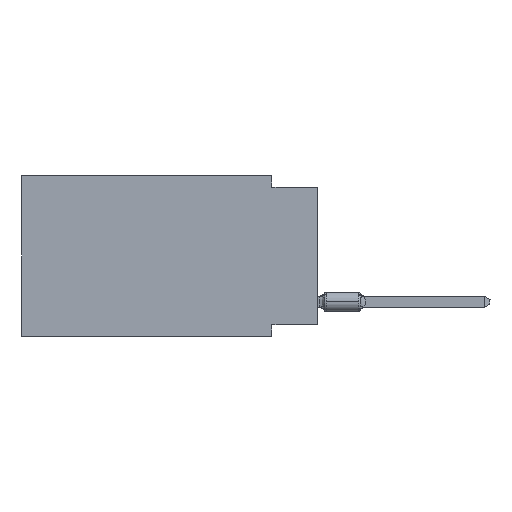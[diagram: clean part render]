
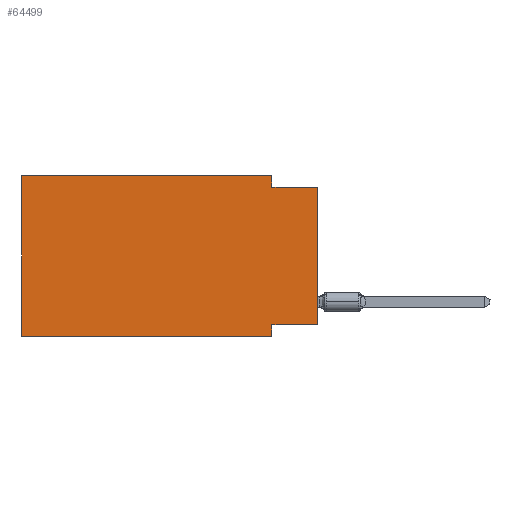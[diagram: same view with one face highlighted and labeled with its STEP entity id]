
A CAD part, left-side view. The second image highlights one B-rep face of the part: STEP entity #64499.
In plain terms, the highlighted planar face has unit normal (-1, 0, 0).
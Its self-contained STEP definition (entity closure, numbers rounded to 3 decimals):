
#1367 = CARTESIAN_POINT ( 'NONE',  ( 0., 16.383, 0. ) ) ;
#1848 = CARTESIAN_POINT ( 'NONE',  ( 0., 16.383, 0. ) ) ;
#3605 = VECTOR ( 'NONE', #41586, 1000. ) ;
#5541 = ORIENTED_EDGE ( 'NONE', *, *, #23059, .T. ) ;
#5818 = LINE ( 'NONE', #66674, #12349 ) ;
#6255 = LINE ( 'NONE', #52389, #24278 ) ;
#6706 = DIRECTION ( 'NONE',  ( 0., 0., 1. ) ) ;
#9025 = CARTESIAN_POINT ( 'NONE',  ( 0., 2.54, 0. ) ) ;
#10659 = EDGE_CURVE ( 'NONE', #60522, #26659, #27059, .T. ) ;
#12349 = VECTOR ( 'NONE', #78007, 1000. ) ;
#13057 = LINE ( 'NONE', #60876, #57707 ) ;
#13425 = VECTOR ( 'NONE', #55308, 1000. ) ;
#15426 = CARTESIAN_POINT ( 'NONE',  ( 0., 0., -8.255 ) ) ;
#16451 = ORIENTED_EDGE ( 'NONE', *, *, #61901, .F. ) ;
#17697 = CARTESIAN_POINT ( 'NONE',  ( 0., 16.383, 0. ) ) ;
#18842 = EDGE_CURVE ( 'NONE', #26659, #22340, #69042, .T. ) ;
#20145 = DIRECTION ( 'NONE',  ( 0., -1., 0. ) ) ;
#22340 = VERTEX_POINT ( 'NONE', #9025 ) ;
#23059 = EDGE_CURVE ( 'NONE', #24144, #85469, #40211, .T. ) ;
#24144 = VERTEX_POINT ( 'NONE', #15426 ) ;
#24278 = VECTOR ( 'NONE', #20145, 1000. ) ;
#26659 = VERTEX_POINT ( 'NONE', #17697 ) ;
#27059 = LINE ( 'NONE', #1367, #13425 ) ;
#28385 = FACE_OUTER_BOUND ( 'NONE', #82070, .T. ) ;
#29486 = CARTESIAN_POINT ( 'NONE',  ( 0., 16.383, 0. ) ) ;
#30424 = EDGE_CURVE ( 'NONE', #35867, #85469, #6255, .T. ) ;
#33253 = CARTESIAN_POINT ( 'NONE',  ( 0., 0., 0. ) ) ;
#35867 = VERTEX_POINT ( 'NONE', #68043 ) ;
#36164 = EDGE_CURVE ( 'NONE', #22340, #35867, #5818, .T. ) ;
#40178 = PLANE ( 'NONE',  #59316 ) ;
#40211 = LINE ( 'NONE', #33253, #54116 ) ;
#41586 = DIRECTION ( 'NONE',  ( 0., 1., 0. ) ) ;
#42982 = DIRECTION ( 'NONE',  ( 0., -1., 0. ) ) ;
#43718 = ORIENTED_EDGE ( 'NONE', *, *, #30424, .F. ) ;
#46697 = DIRECTION ( 'NONE',  ( 0., 0., -1. ) ) ;
#47954 = ORIENTED_EDGE ( 'NONE', *, *, #18842, .F. ) ;
#48053 = CARTESIAN_POINT ( 'NONE',  ( 0., 2.54, -8.89 ) ) ;
#49125 = LINE ( 'NONE', #82144, #53630 ) ;
#49974 = ORIENTED_EDGE ( 'NONE', *, *, #36164, .F. ) ;
#50841 = VERTEX_POINT ( 'NONE', #65071 ) ;
#52389 = CARTESIAN_POINT ( 'NONE',  ( 0., 0., -0.635 ) ) ;
#53630 = VECTOR ( 'NONE', #69506, 1000. ) ;
#54116 = VECTOR ( 'NONE', #6706, 1000. ) ;
#55308 = DIRECTION ( 'NONE',  ( 0., 0., 1. ) ) ;
#56808 = VERTEX_POINT ( 'NONE', #48053 ) ;
#57707 = VECTOR ( 'NONE', #74334, 1000. ) ;
#59316 = AXIS2_PLACEMENT_3D ( 'NONE', #1848, #73196, #46697 ) ;
#60522 = VERTEX_POINT ( 'NONE', #67121 ) ;
#60876 = CARTESIAN_POINT ( 'NONE',  ( 0., 2.54, -8.89 ) ) ;
#61901 = EDGE_CURVE ( 'NONE', #24144, #50841, #74608, .T. ) ;
#62268 = ORIENTED_EDGE ( 'NONE', *, *, #10659, .F. ) ;
#64037 = CARTESIAN_POINT ( 'NONE',  ( 0., 0., -0.635 ) ) ;
#64499 = ADVANCED_FACE ( 'NONE', ( #28385 ), #40178, .F. ) ;
#64721 = VECTOR ( 'NONE', #42982, 1000. ) ;
#65071 = CARTESIAN_POINT ( 'NONE',  ( 0., 2.54, -8.255 ) ) ;
#66674 = CARTESIAN_POINT ( 'NONE',  ( 0., 2.54, 0. ) ) ;
#67121 = CARTESIAN_POINT ( 'NONE',  ( 0., 16.383, -8.89 ) ) ;
#67280 = ORIENTED_EDGE ( 'NONE', *, *, #69987, .F. ) ;
#68043 = CARTESIAN_POINT ( 'NONE',  ( 0., 2.54, -0.635 ) ) ;
#68514 = CARTESIAN_POINT ( 'NONE',  ( 0., 0., -8.255 ) ) ;
#69042 = LINE ( 'NONE', #29486, #64721 ) ;
#69506 = DIRECTION ( 'NONE',  ( 0., -1., 0. ) ) ;
#69987 = EDGE_CURVE ( 'NONE', #50841, #56808, #13057, .T. ) ;
#72381 = EDGE_CURVE ( 'NONE', #60522, #56808, #49125, .T. ) ;
#73196 = DIRECTION ( 'NONE',  ( 1., 0., 0. ) ) ;
#74334 = DIRECTION ( 'NONE',  ( 0., 0., -1. ) ) ;
#74608 = LINE ( 'NONE', #68514, #3605 ) ;
#78007 = DIRECTION ( 'NONE',  ( 0., 0., -1. ) ) ;
#82070 = EDGE_LOOP ( 'NONE', ( #5541, #43718, #49974, #47954, #62268, #85013, #67280, #16451 ) ) ;
#82144 = CARTESIAN_POINT ( 'NONE',  ( 0., 16.383, -8.89 ) ) ;
#85013 = ORIENTED_EDGE ( 'NONE', *, *, #72381, .T. ) ;
#85469 = VERTEX_POINT ( 'NONE', #64037 ) ;
